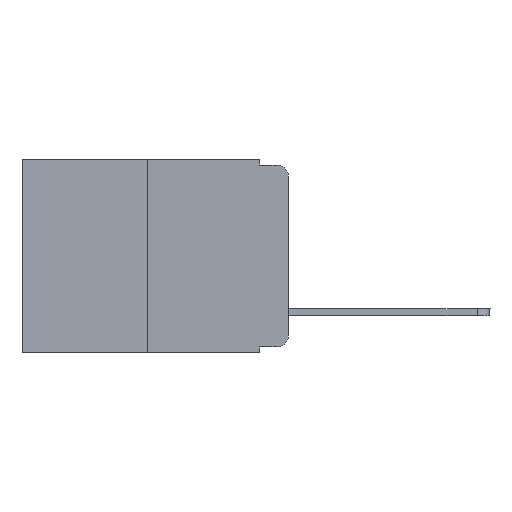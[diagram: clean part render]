
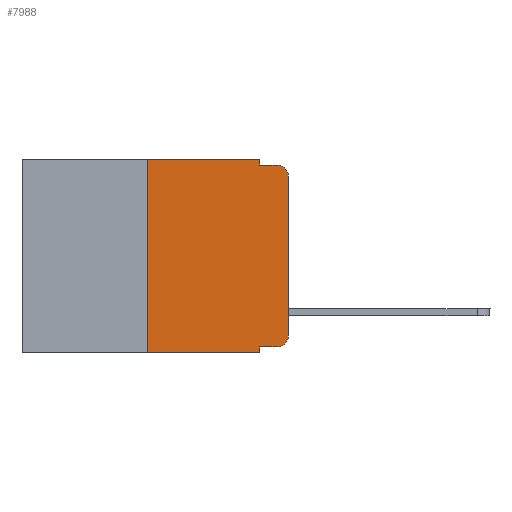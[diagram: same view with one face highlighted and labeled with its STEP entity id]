
A CAD part, left-side view. The second image highlights one B-rep face of the part: STEP entity #7988.
In plain terms, the highlighted planar face has unit normal (-1, 0, 0).
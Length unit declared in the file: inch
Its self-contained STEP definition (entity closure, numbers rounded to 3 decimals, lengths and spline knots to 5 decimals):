
#128 = EDGE_CURVE ( 'NONE', #17719, #5658, #4821, .T. ) ;
#395 = LINE ( 'NONE', #15025, #13039 ) ;
#481 = VECTOR ( 'NONE', #18337, 39.37008 ) ;
#596 = CARTESIAN_POINT ( 'NONE',  ( 0., 0.051, 0. ) ) ;
#1063 = VERTEX_POINT ( 'NONE', #14665 ) ;
#1224 = VERTEX_POINT ( 'NONE', #9604 ) ;
#1445 = VECTOR ( 'NONE', #17909, 39.37008 ) ;
#1489 = DIRECTION ( 'NONE',  ( 0., 0., -1. ) ) ;
#1630 = CARTESIAN_POINT ( 'NONE',  ( 0., 0.02, -0.03 ) ) ;
#1680 = CARTESIAN_POINT ( 'NONE',  ( 0., 0., 0. ) ) ;
#2233 = VERTEX_POINT ( 'NONE', #10496 ) ;
#2441 = FACE_OUTER_BOUND ( 'NONE', #5127, .T. ) ;
#2891 = VERTEX_POINT ( 'NONE', #10752 ) ;
#3157 = DIRECTION ( 'NONE',  ( 0., 0., -1. ) ) ;
#3283 = DIRECTION ( 'NONE',  ( -1., 0., 0. ) ) ;
#3764 = VECTOR ( 'NONE', #17426, 39.37008 ) ;
#4207 = EDGE_CURVE ( 'NONE', #17139, #1224, #20376, .T. ) ;
#4395 = VERTEX_POINT ( 'NONE', #13185 ) ;
#4636 = DIRECTION ( 'NONE',  ( 1., 0., 0. ) ) ;
#4743 = CARTESIAN_POINT ( 'NONE',  ( 0., 0.25, -0.343 ) ) ;
#4798 = EDGE_CURVE ( 'NONE', #17719, #4395, #6990, .T. ) ;
#4821 = LINE ( 'NONE', #18775, #3764 ) ;
#5127 = EDGE_LOOP ( 'NONE', ( #14957, #15102, #18779, #9638, #13487, #18643, #5906, #13668, #13250, #9727 ) ) ;
#5323 = LINE ( 'NONE', #1680, #6088 ) ;
#5658 = VERTEX_POINT ( 'NONE', #14236 ) ;
#5906 = ORIENTED_EDGE ( 'NONE', *, *, #128, .T. ) ;
#6088 = VECTOR ( 'NONE', #9988, 39.37008 ) ;
#6419 = DIRECTION ( 'NONE',  ( 0., 0., -1. ) ) ;
#6501 = PLANE ( 'NONE',  #11701 ) ;
#6990 = LINE ( 'NONE', #14668, #12133 ) ;
#7666 = EDGE_CURVE ( 'NONE', #2233, #14801, #395, .T. ) ;
#7984 = CARTESIAN_POINT ( 'NONE',  ( 0., 0.051, -0.333 ) ) ;
#7988 = ADVANCED_FACE ( 'NONE', ( #2441 ), #6501, .F. ) ;
#9402 = AXIS2_PLACEMENT_3D ( 'NONE', #1630, #3283, #1489 ) ;
#9604 = CARTESIAN_POINT ( 'NONE',  ( 0., 0., -0.313 ) ) ;
#9638 = ORIENTED_EDGE ( 'NONE', *, *, #7666, .F. ) ;
#9727 = ORIENTED_EDGE ( 'NONE', *, *, #4207, .T. ) ;
#9988 = DIRECTION ( 'NONE',  ( 0., 0., 1. ) ) ;
#10025 = DIRECTION ( 'NONE',  ( 0., -1., 0. ) ) ;
#10441 = EDGE_CURVE ( 'NONE', #1063, #5658, #20074, .T. ) ;
#10496 = CARTESIAN_POINT ( 'NONE',  ( 0., 0.051, 0. ) ) ;
#10752 = CARTESIAN_POINT ( 'NONE',  ( 0., 0., -0.03 ) ) ;
#11308 = CARTESIAN_POINT ( 'NONE',  ( 0., 0.02, -0.313 ) ) ;
#11341 = VECTOR ( 'NONE', #6419, 39.37008 ) ;
#11513 = EDGE_CURVE ( 'NONE', #2891, #17809, #16935, .T. ) ;
#11527 = CARTESIAN_POINT ( 'NONE',  ( 0., 0.051, -0.01 ) ) ;
#11701 = AXIS2_PLACEMENT_3D ( 'NONE', #19508, #4636, #19366 ) ;
#11852 = DIRECTION ( 'NONE',  ( 0., 0., -1. ) ) ;
#12133 = VECTOR ( 'NONE', #17828, 39.37008 ) ;
#12170 = VECTOR ( 'NONE', #10025, 39.37008 ) ;
#12276 = LINE ( 'NONE', #7984, #1445 ) ;
#12730 = CARTESIAN_POINT ( 'NONE',  ( 0., 0.051, -0.01 ) ) ;
#13039 = VECTOR ( 'NONE', #11852, 39.37008 ) ;
#13185 = CARTESIAN_POINT ( 'NONE',  ( 0., 0.25, 0. ) ) ;
#13250 = ORIENTED_EDGE ( 'NONE', *, *, #19489, .T. ) ;
#13487 = ORIENTED_EDGE ( 'NONE', *, *, #14397, .F. ) ;
#13668 = ORIENTED_EDGE ( 'NONE', *, *, #10441, .F. ) ;
#14236 = CARTESIAN_POINT ( 'NONE',  ( 0., 0.051, -0.343 ) ) ;
#14397 = EDGE_CURVE ( 'NONE', #4395, #2233, #21160, .T. ) ;
#14398 = DIRECTION ( 'NONE',  ( -1., 0., 0. ) ) ;
#14665 = CARTESIAN_POINT ( 'NONE',  ( 0., 0.051, -0.333 ) ) ;
#14668 = CARTESIAN_POINT ( 'NONE',  ( 0., 0.25, 0. ) ) ;
#14705 = CARTESIAN_POINT ( 'NONE',  ( 0., 0.02, -0.333 ) ) ;
#14765 = CARTESIAN_POINT ( 'NONE',  ( 0., 0.473, 0. ) ) ;
#14801 = VERTEX_POINT ( 'NONE', #12730 ) ;
#14957 = ORIENTED_EDGE ( 'NONE', *, *, #18456, .T. ) ;
#15025 = CARTESIAN_POINT ( 'NONE',  ( 0., 0.051, 0. ) ) ;
#15102 = ORIENTED_EDGE ( 'NONE', *, *, #11513, .T. ) ;
#15422 = LINE ( 'NONE', #11527, #481 ) ;
#15506 = AXIS2_PLACEMENT_3D ( 'NONE', #11308, #14398, #3157 ) ;
#16935 = CIRCLE ( 'NONE', #9402, 0.02 ) ;
#17139 = VERTEX_POINT ( 'NONE', #14705 ) ;
#17201 = EDGE_CURVE ( 'NONE', #14801, #17809, #15422, .T. ) ;
#17426 = DIRECTION ( 'NONE',  ( 0., -1., 0. ) ) ;
#17719 = VERTEX_POINT ( 'NONE', #4743 ) ;
#17809 = VERTEX_POINT ( 'NONE', #19823 ) ;
#17828 = DIRECTION ( 'NONE',  ( 0., 0., 1. ) ) ;
#17909 = DIRECTION ( 'NONE',  ( 0., -1., 0. ) ) ;
#18337 = DIRECTION ( 'NONE',  ( 0., -1., 0. ) ) ;
#18456 = EDGE_CURVE ( 'NONE', #1224, #2891, #5323, .T. ) ;
#18643 = ORIENTED_EDGE ( 'NONE', *, *, #4798, .F. ) ;
#18775 = CARTESIAN_POINT ( 'NONE',  ( 0., 0.473, -0.343 ) ) ;
#18779 = ORIENTED_EDGE ( 'NONE', *, *, #17201, .F. ) ;
#19366 = DIRECTION ( 'NONE',  ( 0., 0., -1. ) ) ;
#19489 = EDGE_CURVE ( 'NONE', #1063, #17139, #12276, .T. ) ;
#19508 = CARTESIAN_POINT ( 'NONE',  ( 0., 0.473, 0. ) ) ;
#19823 = CARTESIAN_POINT ( 'NONE',  ( 0., 0.02, -0.01 ) ) ;
#20074 = LINE ( 'NONE', #596, #11341 ) ;
#20376 = CIRCLE ( 'NONE', #15506, 0.02 ) ;
#21160 = LINE ( 'NONE', #14765, #12170 ) ;
